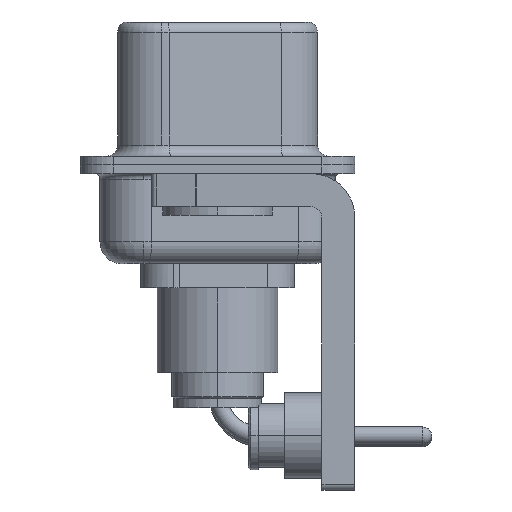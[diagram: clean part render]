
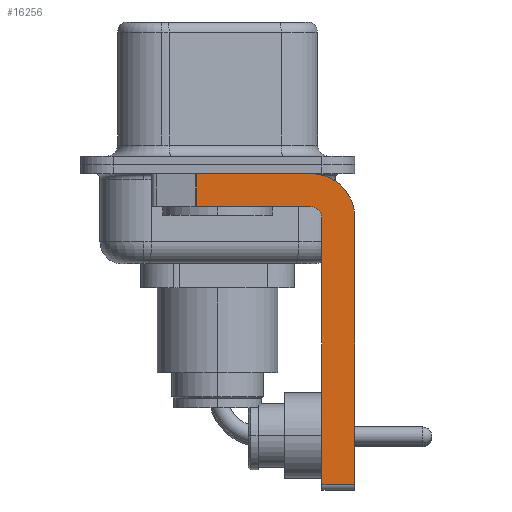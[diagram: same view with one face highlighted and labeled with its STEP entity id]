
A CAD part, left-side view. The second image highlights one B-rep face of the part: STEP entity #16256.
In plain terms, the highlighted planar face has unit normal (-1, 0, 0).
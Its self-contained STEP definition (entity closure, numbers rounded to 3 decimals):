
#208 = CARTESIAN_POINT ( 'NONE',  ( -2.9, -6.25, -14.55 ) ) ;
#395 = CARTESIAN_POINT ( 'NONE',  ( -2.9, 0.978, -1.9 ) ) ;
#794 = DIRECTION ( 'NONE',  ( 1., 0., 0. ) ) ;
#1253 = VERTEX_POINT ( 'NONE', #208 ) ;
#1254 = VERTEX_POINT ( 'NONE', #395 ) ;
#1736 = DIRECTION ( 'NONE',  ( 0., 0., -1. ) ) ;
#1930 = VERTEX_POINT ( 'NONE', #11968 ) ;
#2271 = CARTESIAN_POINT ( 'NONE',  ( -2.9, -4.25, -1.9 ) ) ;
#2560 = CARTESIAN_POINT ( 'NONE',  ( -2.9, 0.978, -1.9 ) ) ;
#2864 = CIRCLE ( 'NONE', #17197, 2. ) ;
#3812 = DIRECTION ( 'NONE',  ( 0., 0., 1. ) ) ;
#4358 = EDGE_CURVE ( 'NONE', #6835, #9097, #11758, .T. ) ;
#4431 = EDGE_CURVE ( 'NONE', #10386, #6835, #19474, .T. ) ;
#4579 = CARTESIAN_POINT ( 'NONE',  ( -2.9, -4.25, -2.4 ) ) ;
#4745 = DIRECTION ( 'NONE',  ( 0., -1., 0. ) ) ;
#4957 = VECTOR ( 'NONE', #16567, 1000. ) ;
#5384 = CARTESIAN_POINT ( 'NONE',  ( -2.9, -4.25, -2.4 ) ) ;
#6708 = ORIENTED_EDGE ( 'NONE', *, *, #11003, .T. ) ;
#6832 = DIRECTION ( 'NONE',  ( 0., 0., 1. ) ) ;
#6835 = VERTEX_POINT ( 'NONE', #15388 ) ;
#6895 = EDGE_CURVE ( 'NONE', #1930, #1254, #16851, .T. ) ;
#6921 = ORIENTED_EDGE ( 'NONE', *, *, #16375, .F. ) ;
#7177 = LINE ( 'NONE', #10216, #10532 ) ;
#7464 = FACE_OUTER_BOUND ( 'NONE', #11808, .T. ) ;
#7490 = AXIS2_PLACEMENT_3D ( 'NONE', #15224, #794, #19921 ) ;
#7661 = DIRECTION ( 'NONE',  ( 0., 0., -1. ) ) ;
#7934 = VERTEX_POINT ( 'NONE', #18886 ) ;
#7992 = ORIENTED_EDGE ( 'NONE', *, *, #4431, .F. ) ;
#9097 = VERTEX_POINT ( 'NONE', #16823 ) ;
#9278 = ORIENTED_EDGE ( 'NONE', *, *, #13551, .F. ) ;
#9731 = CARTESIAN_POINT ( 'NONE',  ( -2.9, -4.75, -14.55 ) ) ;
#9880 = ORIENTED_EDGE ( 'NONE', *, *, #12565, .F. ) ;
#10216 = CARTESIAN_POINT ( 'NONE',  ( -2.9, -4.25, -14.55 ) ) ;
#10238 = EDGE_CURVE ( 'NONE', #1930, #7934, #12671, .T. ) ;
#10386 = VERTEX_POINT ( 'NONE', #9731 ) ;
#10507 = PLANE ( 'NONE',  #7490 ) ;
#10532 = VECTOR ( 'NONE', #18042, 1000. ) ;
#10700 = CARTESIAN_POINT ( 'NONE',  ( -2.9, -6.25, -2.4 ) ) ;
#10919 = ORIENTED_EDGE ( 'NONE', *, *, #6895, .T. ) ;
#11003 = EDGE_CURVE ( 'NONE', #10386, #1253, #7177, .T. ) ;
#11159 = VECTOR ( 'NONE', #19044, 1000. ) ;
#11194 = VERTEX_POINT ( 'NONE', #13640 ) ;
#11737 = DIRECTION ( 'NONE',  ( -1., 0., 0. ) ) ;
#11758 = CIRCLE ( 'NONE', #16763, 0.5 ) ;
#11808 = EDGE_LOOP ( 'NONE', ( #17848, #10919, #9880, #14947, #7992, #6708, #9278, #6921 ) ) ;
#11846 = CARTESIAN_POINT ( 'NONE',  ( -2.9, -4.75, -14.8 ) ) ;
#11968 = CARTESIAN_POINT ( 'NONE',  ( -2.9, 0.978, -0.4 ) ) ;
#12565 = EDGE_CURVE ( 'NONE', #9097, #1254, #18437, .T. ) ;
#12671 = LINE ( 'NONE', #19032, #19243 ) ;
#12777 = VECTOR ( 'NONE', #7661, 1000. ) ;
#13551 = EDGE_CURVE ( 'NONE', #11194, #1253, #14343, .T. ) ;
#13640 = CARTESIAN_POINT ( 'NONE',  ( -2.9, -6.25, -2.4 ) ) ;
#14343 = LINE ( 'NONE', #10700, #11159 ) ;
#14947 = ORIENTED_EDGE ( 'NONE', *, *, #4358, .F. ) ;
#15224 = CARTESIAN_POINT ( 'NONE',  ( -2.9, -4.25, -2.4 ) ) ;
#15388 = CARTESIAN_POINT ( 'NONE',  ( -2.9, -4.75, -2.4 ) ) ;
#16256 = ADVANCED_FACE ( 'NONE', ( #7464 ), #10507, .F. ) ;
#16375 = EDGE_CURVE ( 'NONE', #7934, #11194, #2864, .T. ) ;
#16567 = DIRECTION ( 'NONE',  ( 0., 1., 0. ) ) ;
#16763 = AXIS2_PLACEMENT_3D ( 'NONE', #5384, #11737, #3812 ) ;
#16823 = CARTESIAN_POINT ( 'NONE',  ( -2.9, -4.25, -1.9 ) ) ;
#16851 = LINE ( 'NONE', #2560, #12777 ) ;
#17197 = AXIS2_PLACEMENT_3D ( 'NONE', #4579, #20645, #1736 ) ;
#17848 = ORIENTED_EDGE ( 'NONE', *, *, #10238, .F. ) ;
#18042 = DIRECTION ( 'NONE',  ( 0., -1., 0. ) ) ;
#18081 = VECTOR ( 'NONE', #6832, 1000. ) ;
#18437 = LINE ( 'NONE', #2271, #4957 ) ;
#18886 = CARTESIAN_POINT ( 'NONE',  ( -2.9, -4.25, -0.4 ) ) ;
#19032 = CARTESIAN_POINT ( 'NONE',  ( -2.9, 3., -0.4 ) ) ;
#19044 = DIRECTION ( 'NONE',  ( 0., 0., -1. ) ) ;
#19243 = VECTOR ( 'NONE', #4745, 1000. ) ;
#19474 = LINE ( 'NONE', #11846, #18081 ) ;
#19921 = DIRECTION ( 'NONE',  ( 0., 0., -1. ) ) ;
#20645 = DIRECTION ( 'NONE',  ( 1., 0., 0. ) ) ;
